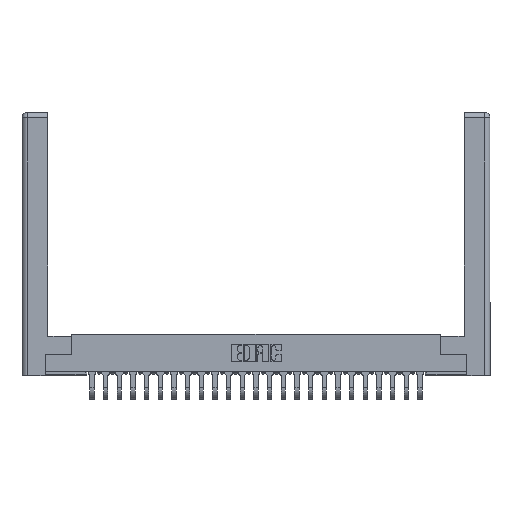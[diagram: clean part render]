
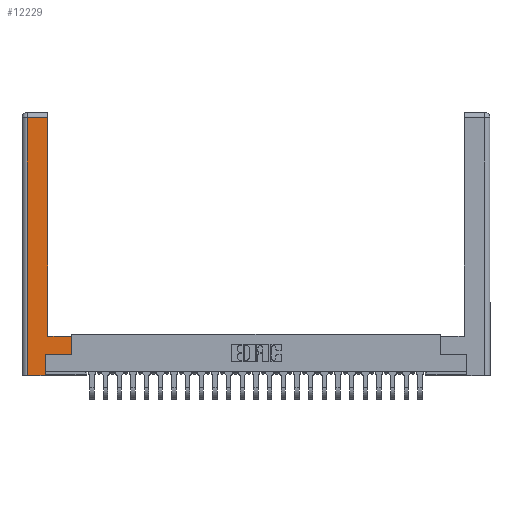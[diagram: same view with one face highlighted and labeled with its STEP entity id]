
A CAD part, top view. The second image highlights one B-rep face of the part: STEP entity #12229.
In plain terms, the highlighted planar face has unit normal (0, 0, 1).
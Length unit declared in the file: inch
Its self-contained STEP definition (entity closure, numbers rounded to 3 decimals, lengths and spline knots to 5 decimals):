
#392 = CARTESIAN_POINT ( 'NONE',  ( 0.565, 0.45, 0. ) ) ;
#597 = LINE ( 'NONE', #8818, #22901 ) ;
#897 = EDGE_CURVE ( 'NONE', #11626, #15990, #18207, .T. ) ;
#962 = DIRECTION ( 'NONE',  ( 1., 0., 0. ) ) ;
#1059 = VERTEX_POINT ( 'NONE', #2111 ) ;
#1148 = DIRECTION ( 'NONE',  ( 0., 0., -1. ) ) ;
#1824 = CARTESIAN_POINT ( 'NONE',  ( 0.565, 0.245, 0. ) ) ;
#2111 = CARTESIAN_POINT ( 'NONE',  ( 0.0615, 2.94, 0. ) ) ;
#2788 = CARTESIAN_POINT ( 'NONE',  ( 0.0615, 0., 0. ) ) ;
#2918 = DIRECTION ( 'NONE',  ( 0., -1., 0. ) ) ;
#3290 = VERTEX_POINT ( 'NONE', #17694 ) ;
#3339 = CARTESIAN_POINT ( 'NONE',  ( 0.295, 2.94, 0. ) ) ;
#3737 = ORIENTED_EDGE ( 'NONE', *, *, #22088, .T. ) ;
#4434 = CARTESIAN_POINT ( 'NONE',  ( 0.295, 0.45, 0. ) ) ;
#4863 = DIRECTION ( 'NONE',  ( 0., 1., 0. ) ) ;
#5204 = ORIENTED_EDGE ( 'NONE', *, *, #20137, .T. ) ;
#5583 = DIRECTION ( 'NONE',  ( 0., 1., 0. ) ) ;
#6879 = FACE_OUTER_BOUND ( 'NONE', #8380, .T. ) ;
#7146 = EDGE_CURVE ( 'NONE', #18961, #22304, #597, .T. ) ;
#7472 = VERTEX_POINT ( 'NONE', #4434 ) ;
#7568 = CARTESIAN_POINT ( 'NONE',  ( 0.565, 0.45, 0. ) ) ;
#7851 = ORIENTED_EDGE ( 'NONE', *, *, #22670, .T. ) ;
#8283 = ORIENTED_EDGE ( 'NONE', *, *, #7146, .T. ) ;
#8380 = EDGE_LOOP ( 'NONE', ( #7851, #22313, #5204, #3737, #8283, #9835, #15823, #14675 ) ) ;
#8818 = CARTESIAN_POINT ( 'NONE',  ( 0.265, 0.245, 0. ) ) ;
#9012 = VERTEX_POINT ( 'NONE', #3339 ) ;
#9274 = CARTESIAN_POINT ( 'NONE',  ( 0.0615, 2.94, 0. ) ) ;
#9835 = ORIENTED_EDGE ( 'NONE', *, *, #17319, .T. ) ;
#10844 = VECTOR ( 'NONE', #5583, 39.37008 ) ;
#10871 = PLANE ( 'NONE',  #20335 ) ;
#11564 = CARTESIAN_POINT ( 'NONE',  ( 0.295, 3., 0. ) ) ;
#11626 = VERTEX_POINT ( 'NONE', #15486 ) ;
#11917 = VECTOR ( 'NONE', #15832, 39.37008 ) ;
#11942 = LINE ( 'NONE', #1824, #24346 ) ;
#12229 = ADVANCED_FACE ( 'NONE', ( #6879 ), #10871, .F. ) ;
#12808 = VECTOR ( 'NONE', #962, 39.37008 ) ;
#12992 = CARTESIAN_POINT ( 'NONE',  ( 0.295, 0.45, 0. ) ) ;
#13008 = CARTESIAN_POINT ( 'NONE',  ( 0., 0., 0. ) ) ;
#13230 = VECTOR ( 'NONE', #23935, 39.37008 ) ;
#13656 = CARTESIAN_POINT ( 'NONE',  ( 0.265, 0., 0. ) ) ;
#14675 = ORIENTED_EDGE ( 'NONE', *, *, #18939, .T. ) ;
#14995 = LINE ( 'NONE', #12992, #23313 ) ;
#15130 = DIRECTION ( 'NONE',  ( -1., 0., 0. ) ) ;
#15486 = CARTESIAN_POINT ( 'NONE',  ( 0.565, 0.245, 0. ) ) ;
#15819 = LINE ( 'NONE', #9274, #13230 ) ;
#15823 = ORIENTED_EDGE ( 'NONE', *, *, #897, .T. ) ;
#15832 = DIRECTION ( 'NONE',  ( 0., 1., 0. ) ) ;
#15990 = VERTEX_POINT ( 'NONE', #392 ) ;
#16085 = EDGE_CURVE ( 'NONE', #9012, #1059, #15819, .T. ) ;
#16637 = CARTESIAN_POINT ( 'NONE',  ( 0.265, 0.245, 0. ) ) ;
#17319 = EDGE_CURVE ( 'NONE', #22304, #11626, #11942, .T. ) ;
#17694 = CARTESIAN_POINT ( 'NONE',  ( 0.0615, 0., 0. ) ) ;
#17761 = DIRECTION ( 'NONE',  ( -1., 0., 0. ) ) ;
#18207 = LINE ( 'NONE', #7568, #10844 ) ;
#18939 = EDGE_CURVE ( 'NONE', #15990, #7472, #14995, .T. ) ;
#18961 = VERTEX_POINT ( 'NONE', #13656 ) ;
#19191 = CARTESIAN_POINT ( 'NONE',  ( 0.265, 0., 0. ) ) ;
#20137 = EDGE_CURVE ( 'NONE', #1059, #3290, #21021, .T. ) ;
#20335 = AXIS2_PLACEMENT_3D ( 'NONE', #13008, #1148, #15130 ) ;
#21021 = LINE ( 'NONE', #2788, #24191 ) ;
#21679 = LINE ( 'NONE', #11564, #11917 ) ;
#22059 = DIRECTION ( 'NONE',  ( 1., 0., 0. ) ) ;
#22088 = EDGE_CURVE ( 'NONE', #3290, #18961, #25303, .T. ) ;
#22304 = VERTEX_POINT ( 'NONE', #16637 ) ;
#22313 = ORIENTED_EDGE ( 'NONE', *, *, #16085, .T. ) ;
#22670 = EDGE_CURVE ( 'NONE', #7472, #9012, #21679, .T. ) ;
#22901 = VECTOR ( 'NONE', #4863, 39.37008 ) ;
#23313 = VECTOR ( 'NONE', #17761, 39.37008 ) ;
#23935 = DIRECTION ( 'NONE',  ( -1., 0., 0. ) ) ;
#24191 = VECTOR ( 'NONE', #2918, 39.37008 ) ;
#24346 = VECTOR ( 'NONE', #22059, 39.37008 ) ;
#25303 = LINE ( 'NONE', #19191, #12808 ) ;
